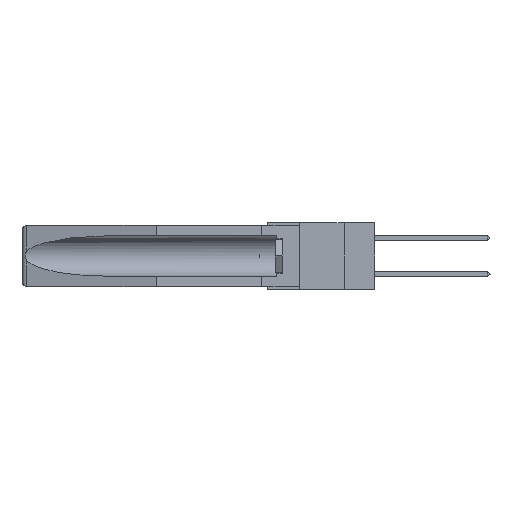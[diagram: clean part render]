
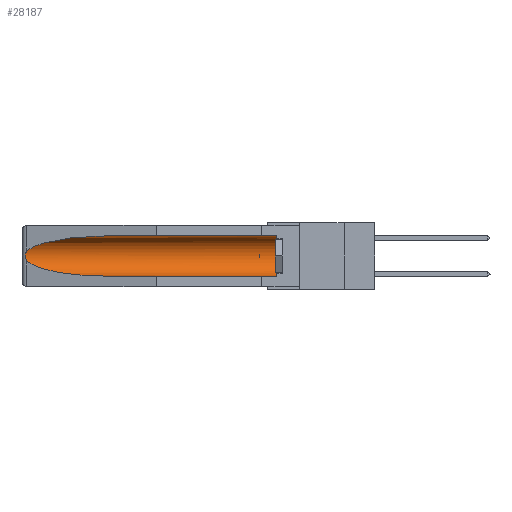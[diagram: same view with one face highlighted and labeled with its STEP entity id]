
A CAD part, left-side view. The second image highlights one B-rep face of the part: STEP entity #28187.
In plain terms, the highlighted cylindrical face has radius 2.857 mm (diameter 5.715 mm), a partial arc.
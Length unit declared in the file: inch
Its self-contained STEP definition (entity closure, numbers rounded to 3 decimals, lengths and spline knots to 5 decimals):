
#1096 =( BOUNDED_CURVE ( )  B_SPLINE_CURVE ( 3, ( #1146, #34130, #28367, #6662 ),
 .UNSPECIFIED., .F., .T. ) 
 B_SPLINE_CURVE_WITH_KNOTS ( ( 4, 4 ),
 ( 4.71239, 6.08839 ),
 .UNSPECIFIED. ) 
 CURVE ( )  GEOMETRIC_REPRESENTATION_ITEM ( )  RATIONAL_B_SPLINE_CURVE ( ( 1., 0.848, 0.848, 1. ) ) 
 REPRESENTATION_ITEM ( '' )  );
#1146 = CARTESIAN_POINT ( 'NONE',  ( 0.155, 1.07973, -0.059 ) ) ;
#2239 = CARTESIAN_POINT ( 'NONE',  ( 0.155, 1.07973, -0.284 ) ) ;
#2259 = CARTESIAN_POINT ( 'NONE',  ( 0.26537, 1.52718, -0.14972 ) ) ;
#2832 = B_SPLINE_CURVE_WITH_KNOTS ( 'NONE', 3,
 ( #2259, #12816, #32233, #15599, #5004, #7529, #7771, #7413, #27137, #10545 ),
 .UNSPECIFIED., .F., .F.,
 ( 4, 2, 2, 2, 4 ),
 ( 0., 0.00029, 0.00058, 0.00087, 0.00117 ),
 .UNSPECIFIED. ) ;
#4122 = DIRECTION ( 'NONE',  ( 0., 1., 0. ) ) ;
#4803 = VERTEX_POINT ( 'NONE', #7989 ) ;
#5004 = CARTESIAN_POINT ( 'NONE',  ( 0.2675, 1.53308, -0.16763 ) ) ;
#5235 = VERTEX_POINT ( 'NONE', #22642 ) ;
#6662 = CARTESIAN_POINT ( 'NONE',  ( 0.26537, 1.52718, -0.14972 ) ) ;
#7413 = CARTESIAN_POINT ( 'NONE',  ( 0.26655, 1.53094, -0.18657 ) ) ;
#7529 = CARTESIAN_POINT ( 'NONE',  ( 0.2675, 1.53308, -0.17534 ) ) ;
#7771 = CARTESIAN_POINT ( 'NONE',  ( 0.2673, 1.53269, -0.17917 ) ) ;
#7989 = CARTESIAN_POINT ( 'NONE',  ( 0.26537, 1.52718, -0.19328 ) ) ;
#8211 = ORIENTED_EDGE ( 'NONE', *, *, #16991, .F. ) ;
#10350 = CARTESIAN_POINT ( 'NONE',  ( 0.155, 0.126, -0.284 ) ) ;
#10545 = CARTESIAN_POINT ( 'NONE',  ( 0.26537, 1.52718, -0.19328 ) ) ;
#10622 = CARTESIAN_POINT ( 'NONE',  ( 0.155, -0.30754, -0.059 ) ) ;
#11134 = FACE_OUTER_BOUND ( 'NONE', #13150, .T. ) ;
#11342 = DIRECTION ( 'NONE',  ( 0., 0., 1. ) ) ;
#11627 = AXIS2_PLACEMENT_3D ( 'NONE', #22356, #30370, #27600 ) ;
#12816 = CARTESIAN_POINT ( 'NONE',  ( 0.26597, 1.52961, -0.15275 ) ) ;
#13150 = EDGE_LOOP ( 'NONE', ( #28108, #27030, #20586, #8211, #33324, #23460 ) ) ;
#13257 = EDGE_CURVE ( 'NONE', #30385, #4803, #2832, .T. ) ;
#15599 = CARTESIAN_POINT ( 'NONE',  ( 0.2673, 1.5327, -0.16383 ) ) ;
#15884 = CYLINDRICAL_SURFACE ( 'NONE', #11627, 0.1125 ) ;
#16547 = CARTESIAN_POINT ( 'NONE',  ( 0.25451, 1.48313, -0.24835 ) ) ;
#16791 = EDGE_CURVE ( 'NONE', #5235, #30385, #1096, .T. ) ;
#16991 = EDGE_CURVE ( 'NONE', #19714, #23329, #20320, .T. ) ;
#17109 = LINE ( 'NONE', #10622, #22314 ) ;
#19113 = CARTESIAN_POINT ( 'NONE',  ( 0.155, 1.07973, -0.284 ) ) ;
#19494 = DIRECTION ( 'NONE',  ( 0., -1., 0. ) ) ;
#19714 = VERTEX_POINT ( 'NONE', #10350 ) ;
#20320 = LINE ( 'NONE', #31727, #34632 ) ;
#20586 = ORIENTED_EDGE ( 'NONE', *, *, #35522, .T. ) ;
#22314 = VECTOR ( 'NONE', #30113, 39.37008 ) ;
#22356 = CARTESIAN_POINT ( 'NONE',  ( 0.155, -0.30754, -0.1715 ) ) ;
#22432 = VERTEX_POINT ( 'NONE', #31607 ) ;
#22642 = CARTESIAN_POINT ( 'NONE',  ( 0.155, 1.07973, -0.059 ) ) ;
#23329 = VERTEX_POINT ( 'NONE', #2239 ) ;
#23372 = EDGE_CURVE ( 'NONE', #19714, #22432, #26790, .T. ) ;
#23460 = ORIENTED_EDGE ( 'NONE', *, *, #32506, .T. ) ;
#26327 =( BOUNDED_CURVE ( )  B_SPLINE_CURVE ( 3, ( #30215, #16547, #32893, #19113 ),
 .UNSPECIFIED., .F., .F. ) 
 B_SPLINE_CURVE_WITH_KNOTS ( ( 4, 4 ),
 ( 0.1948, 1.5708 ),
 .UNSPECIFIED. ) 
 CURVE ( )  GEOMETRIC_REPRESENTATION_ITEM ( )  RATIONAL_B_SPLINE_CURVE ( ( 1., 0.848, 0.848, 1. ) ) 
 REPRESENTATION_ITEM ( '' )  );
#26790 = CIRCLE ( 'NONE', #28296, 0.1125 ) ;
#26979 = CARTESIAN_POINT ( 'NONE',  ( 0.26537, 1.52718, -0.14972 ) ) ;
#27030 = ORIENTED_EDGE ( 'NONE', *, *, #13257, .T. ) ;
#27137 = CARTESIAN_POINT ( 'NONE',  ( 0.26597, 1.5296, -0.19026 ) ) ;
#27600 = DIRECTION ( 'NONE',  ( 0., 0., 1. ) ) ;
#27953 = CARTESIAN_POINT ( 'NONE',  ( 0.155, 0.126, -0.1715 ) ) ;
#28108 = ORIENTED_EDGE ( 'NONE', *, *, #16791, .T. ) ;
#28187 = ADVANCED_FACE ( 'NONE', ( #11134 ), #15884, .F. ) ;
#28296 = AXIS2_PLACEMENT_3D ( 'NONE', #27953, #19494, #11342 ) ;
#28367 = CARTESIAN_POINT ( 'NONE',  ( 0.25451, 1.48313, -0.09465 ) ) ;
#30113 = DIRECTION ( 'NONE',  ( 0., 1., 0. ) ) ;
#30215 = CARTESIAN_POINT ( 'NONE',  ( 0.26537, 1.52718, -0.19328 ) ) ;
#30370 = DIRECTION ( 'NONE',  ( 0., 1., 0. ) ) ;
#30385 = VERTEX_POINT ( 'NONE', #26979 ) ;
#31607 = CARTESIAN_POINT ( 'NONE',  ( 0.155, 0.126, -0.059 ) ) ;
#31727 = CARTESIAN_POINT ( 'NONE',  ( 0.155, -0.30754, -0.284 ) ) ;
#32233 = CARTESIAN_POINT ( 'NONE',  ( 0.26654, 1.53092, -0.15636 ) ) ;
#32506 = EDGE_CURVE ( 'NONE', #22432, #5235, #17109, .T. ) ;
#32893 = CARTESIAN_POINT ( 'NONE',  ( 0.21114, 1.30732, -0.284 ) ) ;
#33324 = ORIENTED_EDGE ( 'NONE', *, *, #23372, .T. ) ;
#34130 = CARTESIAN_POINT ( 'NONE',  ( 0.21114, 1.30732, -0.059 ) ) ;
#34632 = VECTOR ( 'NONE', #4122, 39.37008 ) ;
#35522 = EDGE_CURVE ( 'NONE', #4803, #23329, #26327, .T. ) ;
